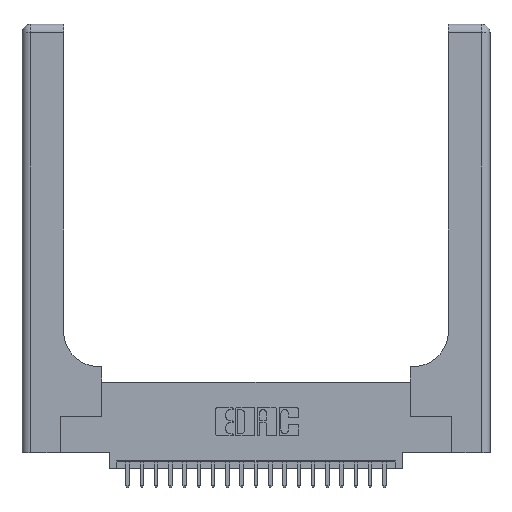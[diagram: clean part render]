
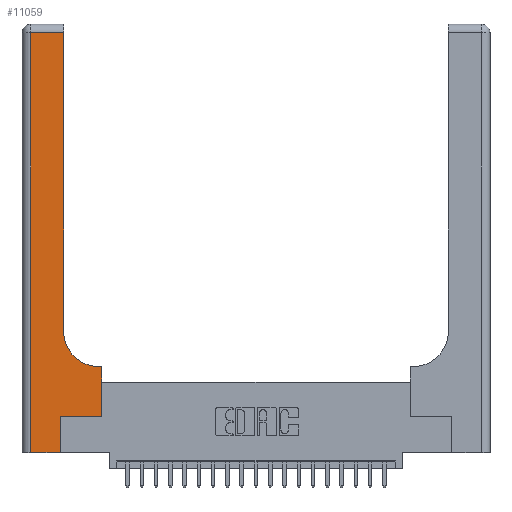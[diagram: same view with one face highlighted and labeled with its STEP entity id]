
A CAD part, top view. The second image highlights one B-rep face of the part: STEP entity #11059.
In plain terms, the highlighted planar face has unit normal (0, 0, 1).
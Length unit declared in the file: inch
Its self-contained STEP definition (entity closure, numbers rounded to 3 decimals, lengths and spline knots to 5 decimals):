
#154 = EDGE_CURVE ( 'NONE', #5976, #8803, #2417, .T. ) ;
#420 = ORIENTED_EDGE ( 'NONE', *, *, #154, .T. ) ;
#749 = CARTESIAN_POINT ( 'NONE',  ( 0.269, 0., 0.37 ) ) ;
#973 = CARTESIAN_POINT ( 'NONE',  ( 0.5415, 0.6, 0.37 ) ) ;
#1133 = AXIS2_PLACEMENT_3D ( 'NONE', #4819, #6681, #19218 ) ;
#1249 = EDGE_CURVE ( 'NONE', #18267, #5976, #4414, .T. ) ;
#1384 = VECTOR ( 'NONE', #6030, 39.37008 ) ;
#1589 = EDGE_CURVE ( 'NONE', #14169, #12321, #21476, .T. ) ;
#2417 = LINE ( 'NONE', #12555, #16370 ) ;
#2991 = VERTEX_POINT ( 'NONE', #8260 ) ;
#3119 = ORIENTED_EDGE ( 'NONE', *, *, #1249, .T. ) ;
#3705 = LINE ( 'NONE', #19765, #22247 ) ;
#3917 = EDGE_CURVE ( 'NONE', #2991, #14169, #5479, .T. ) ;
#4414 = LINE ( 'NONE', #6190, #9352 ) ;
#4819 = CARTESIAN_POINT ( 'NONE',  ( 0., 3., 0.37 ) ) ;
#5479 = LINE ( 'NONE', #8746, #10411 ) ;
#5976 = VERTEX_POINT ( 'NONE', #16526 ) ;
#6030 = DIRECTION ( 'NONE',  ( 0., 1., 0. ) ) ;
#6102 = DIRECTION ( 'NONE',  ( -1., 0., 0. ) ) ;
#6190 = CARTESIAN_POINT ( 'NONE',  ( 0., 2.94, 0.37 ) ) ;
#6277 = ORIENTED_EDGE ( 'NONE', *, *, #15714, .T. ) ;
#6681 = DIRECTION ( 'NONE',  ( 0., 0., -1. ) ) ;
#7211 = VECTOR ( 'NONE', #18889, 39.37008 ) ;
#7342 = DIRECTION ( 'NONE',  ( 0., -1., 0. ) ) ;
#7345 = ORIENTED_EDGE ( 'NONE', *, *, #1589, .T. ) ;
#7658 = FACE_OUTER_BOUND ( 'NONE', #11080, .T. ) ;
#8260 = CARTESIAN_POINT ( 'NONE',  ( 0.5585, 0.6, 0.37 ) ) ;
#8746 = CARTESIAN_POINT ( 'NONE',  ( 0.2915, 0.6, 0.37 ) ) ;
#8803 = VERTEX_POINT ( 'NONE', #22341 ) ;
#9019 = ORIENTED_EDGE ( 'NONE', *, *, #3917, .T. ) ;
#9352 = VECTOR ( 'NONE', #6102, 39.37008 ) ;
#9564 = AXIS2_PLACEMENT_3D ( 'NONE', #12543, #12537, #12416 ) ;
#9955 = CARTESIAN_POINT ( 'NONE',  ( 0.269, 0.25, 0.37 ) ) ;
#10411 = VECTOR ( 'NONE', #21095, 39.37008 ) ;
#10412 = ORIENTED_EDGE ( 'NONE', *, *, #12697, .T. ) ;
#10469 = EDGE_CURVE ( 'NONE', #12321, #18267, #10565, .T. ) ;
#10565 = LINE ( 'NONE', #12370, #19937 ) ;
#11059 = ADVANCED_FACE ( 'NONE', ( #7658 ), #15678, .F. ) ;
#11080 = EDGE_LOOP ( 'NONE', ( #16064, #3119, #420, #12526, #6277, #10412, #14196, #9019, #7345 ) ) ;
#12082 = LINE ( 'NONE', #17125, #7211 ) ;
#12321 = VERTEX_POINT ( 'NONE', #18912 ) ;
#12370 = CARTESIAN_POINT ( 'NONE',  ( 0.2915, 3., 0.37 ) ) ;
#12416 = DIRECTION ( 'NONE',  ( 1., 0., 0. ) ) ;
#12526 = ORIENTED_EDGE ( 'NONE', *, *, #12985, .T. ) ;
#12537 = DIRECTION ( 'NONE',  ( 0., 0., -1. ) ) ;
#12543 = CARTESIAN_POINT ( 'NONE',  ( 0.5415, 0.85, 0.37 ) ) ;
#12555 = CARTESIAN_POINT ( 'NONE',  ( 0.06, 3., 0.37 ) ) ;
#12697 = EDGE_CURVE ( 'NONE', #12952, #15693, #3705, .T. ) ;
#12952 = VERTEX_POINT ( 'NONE', #9955 ) ;
#12985 = EDGE_CURVE ( 'NONE', #8803, #23247, #12082, .T. ) ;
#13581 = DIRECTION ( 'NONE',  ( 0., 1., 0. ) ) ;
#14169 = VERTEX_POINT ( 'NONE', #973 ) ;
#14196 = ORIENTED_EDGE ( 'NONE', *, *, #21327, .T. ) ;
#15134 = CARTESIAN_POINT ( 'NONE',  ( 0.5585, 0.25, 0.37 ) ) ;
#15678 = PLANE ( 'NONE',  #1133 ) ;
#15693 = VERTEX_POINT ( 'NONE', #17083 ) ;
#15714 = EDGE_CURVE ( 'NONE', #23247, #12952, #17564, .T. ) ;
#16064 = ORIENTED_EDGE ( 'NONE', *, *, #10469, .T. ) ;
#16370 = VECTOR ( 'NONE', #7342, 39.37008 ) ;
#16526 = CARTESIAN_POINT ( 'NONE',  ( 0.06, 2.94, 0.37 ) ) ;
#17083 = CARTESIAN_POINT ( 'NONE',  ( 0.5585, 0.25, 0.37 ) ) ;
#17125 = CARTESIAN_POINT ( 'NONE',  ( 0., 0., 0.37 ) ) ;
#17564 = LINE ( 'NONE', #749, #22139 ) ;
#18267 = VERTEX_POINT ( 'NONE', #18816 ) ;
#18816 = CARTESIAN_POINT ( 'NONE',  ( 0.2915, 2.94, 0.37 ) ) ;
#18889 = DIRECTION ( 'NONE',  ( 1., 0., 0. ) ) ;
#18912 = CARTESIAN_POINT ( 'NONE',  ( 0.2915, 0.85, 0.37 ) ) ;
#19218 = DIRECTION ( 'NONE',  ( -1., 0., 0. ) ) ;
#19765 = CARTESIAN_POINT ( 'NONE',  ( 0.269, 0.25, 0.37 ) ) ;
#19937 = VECTOR ( 'NONE', #22882, 39.37008 ) ;
#20592 = LINE ( 'NONE', #15134, #1384 ) ;
#21095 = DIRECTION ( 'NONE',  ( -1., 0., 0. ) ) ;
#21327 = EDGE_CURVE ( 'NONE', #15693, #2991, #20592, .T. ) ;
#21476 = CIRCLE ( 'NONE', #9564, 0.25 ) ;
#21506 = DIRECTION ( 'NONE',  ( 1., 0., 0. ) ) ;
#21672 = CARTESIAN_POINT ( 'NONE',  ( 0.269, 0., 0.37 ) ) ;
#22139 = VECTOR ( 'NONE', #13581, 39.37008 ) ;
#22247 = VECTOR ( 'NONE', #21506, 39.37008 ) ;
#22341 = CARTESIAN_POINT ( 'NONE',  ( 0.06, 0., 0.37 ) ) ;
#22882 = DIRECTION ( 'NONE',  ( 0., 1., 0. ) ) ;
#23247 = VERTEX_POINT ( 'NONE', #21672 ) ;
